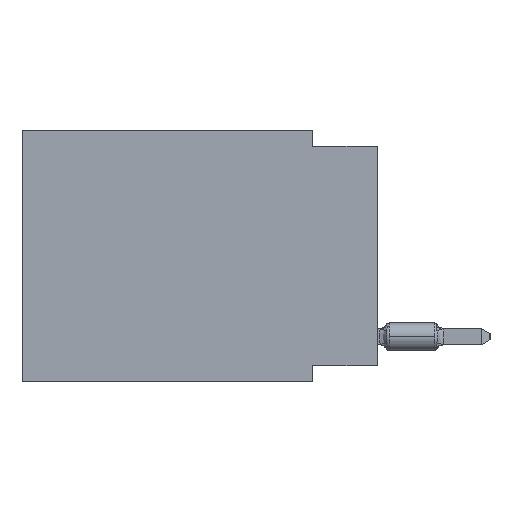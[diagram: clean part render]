
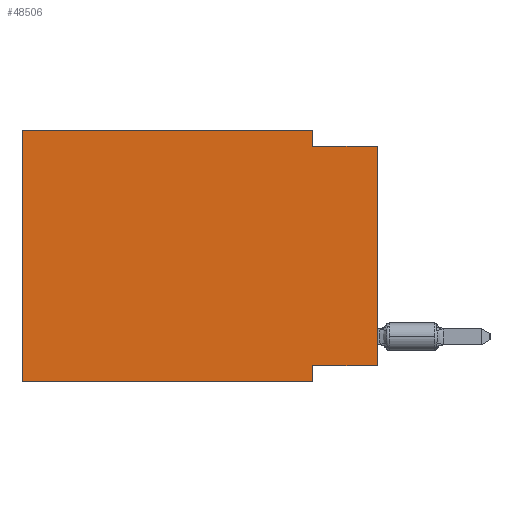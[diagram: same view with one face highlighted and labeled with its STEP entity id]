
A CAD part, left-side view. The second image highlights one B-rep face of the part: STEP entity #48506.
In plain terms, the highlighted planar face has unit normal (-1, 0, 0).
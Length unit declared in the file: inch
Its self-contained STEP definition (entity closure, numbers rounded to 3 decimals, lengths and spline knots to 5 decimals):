
#5337 = LINE ( 'NONE', #37963, #36450 ) ;
#6555 = ORIENTED_EDGE ( 'NONE', *, *, #16745, .F. ) ;
#7084 = EDGE_CURVE ( 'NONE', #7511, #18980, #13027, .T. ) ;
#7391 = LINE ( 'NONE', #31841, #52303 ) ;
#7511 = VERTEX_POINT ( 'NONE', #52825 ) ;
#8390 = DIRECTION ( 'NONE',  ( 0., 0., -1. ) ) ;
#8435 = VECTOR ( 'NONE', #8390, 39.37008 ) ;
#9219 = VERTEX_POINT ( 'NONE', #52147 ) ;
#10266 = ORIENTED_EDGE ( 'NONE', *, *, #20712, .F. ) ;
#10410 = EDGE_CURVE ( 'NONE', #32997, #9219, #5337, .T. ) ;
#10628 = DIRECTION ( 'NONE',  ( 0., 0., -1. ) ) ;
#10669 = CARTESIAN_POINT ( 'NONE',  ( 0., 0.55, -0.39 ) ) ;
#12363 = VECTOR ( 'NONE', #44269, 39.37008 ) ;
#12951 = CARTESIAN_POINT ( 'NONE',  ( 0., 0.1, -0.025 ) ) ;
#13027 = LINE ( 'NONE', #27137, #59265 ) ;
#13209 = ORIENTED_EDGE ( 'NONE', *, *, #10410, .F. ) ;
#15093 = CARTESIAN_POINT ( 'NONE',  ( 0., 0., -0.025 ) ) ;
#15911 = DIRECTION ( 'NONE',  ( 1., 0., 0. ) ) ;
#16004 = AXIS2_PLACEMENT_3D ( 'NONE', #16217, #15911, #35320 ) ;
#16161 = VERTEX_POINT ( 'NONE', #12951 ) ;
#16217 = CARTESIAN_POINT ( 'NONE',  ( 0., 0.55, 0. ) ) ;
#16745 = EDGE_CURVE ( 'NONE', #18980, #55428, #45459, .T. ) ;
#16938 = VECTOR ( 'NONE', #34472, 39.37008 ) ;
#18980 = VERTEX_POINT ( 'NONE', #49250 ) ;
#19562 = DIRECTION ( 'NONE',  ( 0., 0., 1. ) ) ;
#20712 = EDGE_CURVE ( 'NONE', #62020, #32997, #7391, .T. ) ;
#21212 = PLANE ( 'NONE',  #16004 ) ;
#21997 = EDGE_LOOP ( 'NONE', ( #29717, #32337, #32103, #13209, #10266, #56366, #6555, #30343 ) ) ;
#24270 = EDGE_CURVE ( 'NONE', #9219, #16161, #41988, .T. ) ;
#24484 = DIRECTION ( 'NONE',  ( 0., -1., 0. ) ) ;
#27137 = CARTESIAN_POINT ( 'NONE',  ( 0., 0., -0.365 ) ) ;
#29717 = ORIENTED_EDGE ( 'NONE', *, *, #40667, .T. ) ;
#30282 = VECTOR ( 'NONE', #19562, 39.37008 ) ;
#30343 = ORIENTED_EDGE ( 'NONE', *, *, #7084, .F. ) ;
#30722 = VERTEX_POINT ( 'NONE', #15093 ) ;
#31841 = CARTESIAN_POINT ( 'NONE',  ( 0., 0.55, 0. ) ) ;
#32103 = ORIENTED_EDGE ( 'NONE', *, *, #24270, .F. ) ;
#32337 = ORIENTED_EDGE ( 'NONE', *, *, #47992, .F. ) ;
#32453 = DIRECTION ( 'NONE',  ( 0., 1., 0. ) ) ;
#32997 = VERTEX_POINT ( 'NONE', #46540 ) ;
#34466 = CARTESIAN_POINT ( 'NONE',  ( 0., 0.1, -0.39 ) ) ;
#34472 = DIRECTION ( 'NONE',  ( 0., -1., 0. ) ) ;
#35320 = DIRECTION ( 'NONE',  ( 0., 0., -1. ) ) ;
#36450 = VECTOR ( 'NONE', #24484, 39.37008 ) ;
#37963 = CARTESIAN_POINT ( 'NONE',  ( 0., 0.55, 0. ) ) ;
#38069 = CARTESIAN_POINT ( 'NONE',  ( 0., 0., 0. ) ) ;
#40667 = EDGE_CURVE ( 'NONE', #7511, #30722, #53511, .T. ) ;
#40880 = VECTOR ( 'NONE', #10628, 39.37008 ) ;
#41988 = LINE ( 'NONE', #56155, #8435 ) ;
#43760 = EDGE_CURVE ( 'NONE', #62020, #55428, #59040, .T. ) ;
#44269 = DIRECTION ( 'NONE',  ( 0., -1., 0. ) ) ;
#45459 = LINE ( 'NONE', #34466, #40880 ) ;
#46540 = CARTESIAN_POINT ( 'NONE',  ( 0., 0.55, 0. ) ) ;
#47992 = EDGE_CURVE ( 'NONE', #16161, #30722, #58692, .T. ) ;
#48073 = CARTESIAN_POINT ( 'NONE',  ( 0., 0.55, -0.39 ) ) ;
#48506 = ADVANCED_FACE ( 'NONE', ( #50738 ), #21212, .F. ) ;
#48653 = CARTESIAN_POINT ( 'NONE',  ( 0., 0., -0.025 ) ) ;
#49250 = CARTESIAN_POINT ( 'NONE',  ( 0., 0.1, -0.365 ) ) ;
#50738 = FACE_OUTER_BOUND ( 'NONE', #21997, .T. ) ;
#52147 = CARTESIAN_POINT ( 'NONE',  ( 0., 0.1, 0. ) ) ;
#52303 = VECTOR ( 'NONE', #60472, 39.37008 ) ;
#52825 = CARTESIAN_POINT ( 'NONE',  ( 0., 0., -0.365 ) ) ;
#53511 = LINE ( 'NONE', #38069, #30282 ) ;
#55428 = VERTEX_POINT ( 'NONE', #59855 ) ;
#56155 = CARTESIAN_POINT ( 'NONE',  ( 0., 0.1, 0. ) ) ;
#56366 = ORIENTED_EDGE ( 'NONE', *, *, #43760, .T. ) ;
#58692 = LINE ( 'NONE', #48653, #16938 ) ;
#59040 = LINE ( 'NONE', #10669, #12363 ) ;
#59265 = VECTOR ( 'NONE', #32453, 39.37008 ) ;
#59855 = CARTESIAN_POINT ( 'NONE',  ( 0., 0.1, -0.39 ) ) ;
#60472 = DIRECTION ( 'NONE',  ( 0., 0., 1. ) ) ;
#62020 = VERTEX_POINT ( 'NONE', #48073 ) ;
